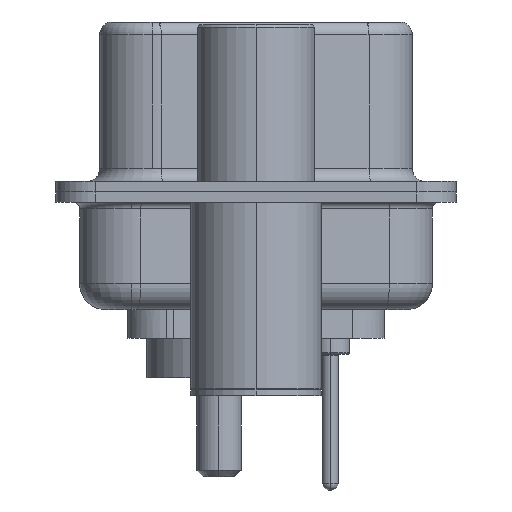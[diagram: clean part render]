
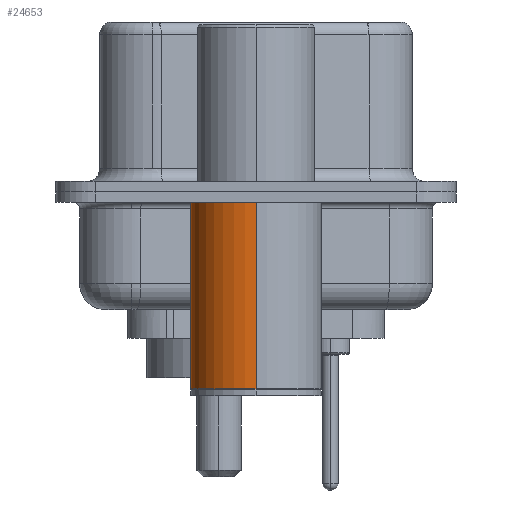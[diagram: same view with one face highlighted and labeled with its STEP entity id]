
A CAD part, left-side view. The second image highlights one B-rep face of the part: STEP entity #24653.
In plain terms, the highlighted cylindrical face has radius 2.5 mm (diameter 5 mm), a partial arc.
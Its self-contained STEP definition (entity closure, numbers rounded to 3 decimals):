
#1911 = DIRECTION ( 'NONE',  ( 0., 0., 1. ) ) ;
#2607 = AXIS2_PLACEMENT_3D ( 'NONE', #21765, #8799, #23954 ) ;
#3263 = DIRECTION ( 'NONE',  ( 1., 0., 0. ) ) ;
#3675 = EDGE_CURVE ( 'NONE', #6287, #17457, #11561, .T. ) ;
#3728 = LINE ( 'NONE', #16107, #20384 ) ;
#4933 = EDGE_LOOP ( 'NONE', ( #24751, #9231, #21526, #5238 ) ) ;
#5238 = ORIENTED_EDGE ( 'NONE', *, *, #22780, .F. ) ;
#6287 = VERTEX_POINT ( 'NONE', #13696 ) ;
#6819 = DIRECTION ( 'NONE',  ( 0., 0., 1. ) ) ;
#8334 = VERTEX_POINT ( 'NONE', #26717 ) ;
#8799 = DIRECTION ( 'NONE',  ( 0., 0., 1. ) ) ;
#8972 = EDGE_CURVE ( 'NONE', #17457, #8334, #3728, .T. ) ;
#9231 = ORIENTED_EDGE ( 'NONE', *, *, #8972, .T. ) ;
#9854 = CARTESIAN_POINT ( 'NONE',  ( 0., 0., 0.581 ) ) ;
#11346 = VERTEX_POINT ( 'NONE', #15475 ) ;
#11561 = CIRCLE ( 'NONE', #14407, 2.5 ) ;
#11644 = CYLINDRICAL_SURFACE ( 'NONE', #12700, 2.5 ) ;
#12700 = AXIS2_PLACEMENT_3D ( 'NONE', #9854, #27237, #3263 ) ;
#13696 = CARTESIAN_POINT ( 'NONE',  ( 2.5, 0., -7.525 ) ) ;
#14407 = AXIS2_PLACEMENT_3D ( 'NONE', #22379, #6819, #15345 ) ;
#14451 = LINE ( 'NONE', #14977, #19550 ) ;
#14977 = CARTESIAN_POINT ( 'NONE',  ( 2.5, 0., 0.581 ) ) ;
#15345 = DIRECTION ( 'NONE',  ( 1., 0., 0. ) ) ;
#15475 = CARTESIAN_POINT ( 'NONE',  ( 2.5, 0., -0.4 ) ) ;
#16107 = CARTESIAN_POINT ( 'NONE',  ( -2.5, 0., 0.581 ) ) ;
#17457 = VERTEX_POINT ( 'NONE', #27322 ) ;
#18271 = DIRECTION ( 'NONE',  ( 0., 0., 1. ) ) ;
#19550 = VECTOR ( 'NONE', #1911, 1000. ) ;
#20384 = VECTOR ( 'NONE', #18271, 1000. ) ;
#21526 = ORIENTED_EDGE ( 'NONE', *, *, #27456, .F. ) ;
#21765 = CARTESIAN_POINT ( 'NONE',  ( 0., 0., -0.4 ) ) ;
#22379 = CARTESIAN_POINT ( 'NONE',  ( 0., 0., -7.525 ) ) ;
#22780 = EDGE_CURVE ( 'NONE', #6287, #11346, #14451, .T. ) ;
#23884 = FACE_OUTER_BOUND ( 'NONE', #4933, .T. ) ;
#23954 = DIRECTION ( 'NONE',  ( 1., 0., 0. ) ) ;
#24653 = ADVANCED_FACE ( 'NONE', ( #23884 ), #11644, .T. ) ;
#24669 = CIRCLE ( 'NONE', #2607, 2.5 ) ;
#24751 = ORIENTED_EDGE ( 'NONE', *, *, #3675, .T. ) ;
#26717 = CARTESIAN_POINT ( 'NONE',  ( -2.5, 0., -0.4 ) ) ;
#27237 = DIRECTION ( 'NONE',  ( 0., 0., 1. ) ) ;
#27322 = CARTESIAN_POINT ( 'NONE',  ( -2.5, 0., -7.525 ) ) ;
#27456 = EDGE_CURVE ( 'NONE', #11346, #8334, #24669, .T. ) ;
